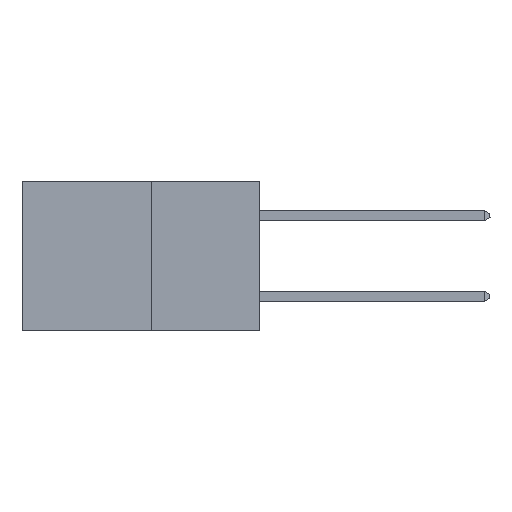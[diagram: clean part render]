
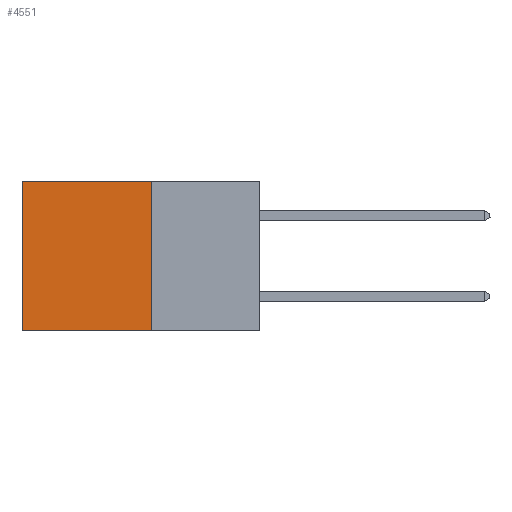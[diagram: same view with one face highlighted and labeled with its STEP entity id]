
A CAD part, left-side view. The second image highlights one B-rep face of the part: STEP entity #4551.
In plain terms, the highlighted planar face has unit normal (-1, 0, 0).
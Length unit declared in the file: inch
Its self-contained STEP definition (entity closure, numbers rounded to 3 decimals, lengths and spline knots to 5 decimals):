
#183 = CARTESIAN_POINT ( 'NONE',  ( 0.277, 0.59, -0.37 ) ) ;
#430 = LINE ( 'NONE', #5553, #17262 ) ;
#568 = DIRECTION ( 'NONE',  ( 0., 1., 0. ) ) ;
#812 = EDGE_LOOP ( 'NONE', ( #10780, #12466, #6502, #6165 ) ) ;
#1308 = CARTESIAN_POINT ( 'NONE',  ( 0.277, 0.27, -0.37 ) ) ;
#1739 = CARTESIAN_POINT ( 'NONE',  ( 0.277, 0.59, 0. ) ) ;
#3207 = CARTESIAN_POINT ( 'NONE',  ( 0.277, 0.27, -0.37 ) ) ;
#3329 = VERTEX_POINT ( 'NONE', #1739 ) ;
#4239 = DIRECTION ( 'NONE',  ( 0., 0., -1. ) ) ;
#4372 = CARTESIAN_POINT ( 'NONE',  ( 0.277, 0.59, -0.37 ) ) ;
#4472 = DIRECTION ( 'NONE',  ( 0., 1., 0. ) ) ;
#4551 = ADVANCED_FACE ( 'NONE', ( #7053 ), #12958, .F. ) ;
#4688 = VECTOR ( 'NONE', #4472, 39.37008 ) ;
#4844 = DIRECTION ( 'NONE',  ( 0., 0., -1. ) ) ;
#4865 = AXIS2_PLACEMENT_3D ( 'NONE', #3207, #5354, #4844 ) ;
#5354 = DIRECTION ( 'NONE',  ( 1., 0., 0. ) ) ;
#5553 = CARTESIAN_POINT ( 'NONE',  ( 0.277, 0.27, -0.37 ) ) ;
#6165 = ORIENTED_EDGE ( 'NONE', *, *, #16621, .T. ) ;
#6502 = ORIENTED_EDGE ( 'NONE', *, *, #19086, .F. ) ;
#6752 = LINE ( 'NONE', #12679, #10686 ) ;
#7053 = FACE_OUTER_BOUND ( 'NONE', #812, .T. ) ;
#9113 = VERTEX_POINT ( 'NONE', #9574 ) ;
#9574 = CARTESIAN_POINT ( 'NONE',  ( 0.277, 0.27, 0. ) ) ;
#10686 = VECTOR ( 'NONE', #4239, 39.37008 ) ;
#10780 = ORIENTED_EDGE ( 'NONE', *, *, #13783, .T. ) ;
#12466 = ORIENTED_EDGE ( 'NONE', *, *, #18952, .F. ) ;
#12679 = CARTESIAN_POINT ( 'NONE',  ( 0.277, 0.27, -0.37 ) ) ;
#12958 = PLANE ( 'NONE',  #4865 ) ;
#13471 = VERTEX_POINT ( 'NONE', #183 ) ;
#13783 = EDGE_CURVE ( 'NONE', #3329, #13471, #14725, .T. ) ;
#14590 = CARTESIAN_POINT ( 'NONE',  ( 0.277, 0.27, 0. ) ) ;
#14725 = LINE ( 'NONE', #4372, #18120 ) ;
#15317 = VERTEX_POINT ( 'NONE', #1308 ) ;
#16621 = EDGE_CURVE ( 'NONE', #9113, #3329, #18126, .T. ) ;
#17262 = VECTOR ( 'NONE', #568, 39.37008 ) ;
#18120 = VECTOR ( 'NONE', #19527, 39.37008 ) ;
#18126 = LINE ( 'NONE', #14590, #4688 ) ;
#18952 = EDGE_CURVE ( 'NONE', #15317, #13471, #430, .T. ) ;
#19086 = EDGE_CURVE ( 'NONE', #9113, #15317, #6752, .T. ) ;
#19527 = DIRECTION ( 'NONE',  ( 0., 0., -1. ) ) ;
